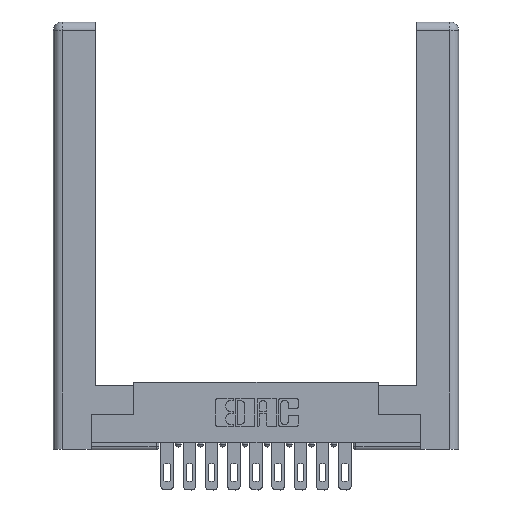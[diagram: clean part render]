
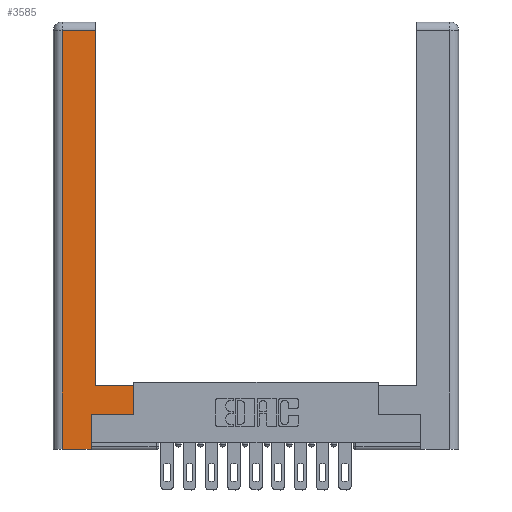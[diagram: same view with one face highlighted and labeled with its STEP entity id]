
A CAD part, top view. The second image highlights one B-rep face of the part: STEP entity #3585.
In plain terms, the highlighted planar face has unit normal (0, 0, 1).
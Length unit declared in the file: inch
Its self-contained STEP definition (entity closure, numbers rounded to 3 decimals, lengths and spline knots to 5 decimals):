
#285 = EDGE_CURVE ( 'NONE', #2528, #12402, #13260, .T. ) ;
#314 = VECTOR ( 'NONE', #14317, 39.37008 ) ;
#324 = DIRECTION ( 'NONE',  ( 0., -1., 0. ) ) ;
#341 = FACE_OUTER_BOUND ( 'NONE', #1421, .T. ) ;
#412 = EDGE_CURVE ( 'NONE', #4392, #11745, #2826, .T. ) ;
#579 = DIRECTION ( 'NONE',  ( -1., 0., 0. ) ) ;
#1043 = CARTESIAN_POINT ( 'NONE',  ( 0.565, 0.45, 0. ) ) ;
#1097 = CARTESIAN_POINT ( 'NONE',  ( 0.265, 0., 0. ) ) ;
#1421 = EDGE_LOOP ( 'NONE', ( #4682, #1939, #2007, #12526, #7499, #11966, #8899, #12150 ) ) ;
#1589 = CARTESIAN_POINT ( 'NONE',  ( 0.565, 0.245, 0. ) ) ;
#1939 = ORIENTED_EDGE ( 'NONE', *, *, #285, .T. ) ;
#2001 = CARTESIAN_POINT ( 'NONE',  ( 0.265, 0.245, 0. ) ) ;
#2007 = ORIENTED_EDGE ( 'NONE', *, *, #9992, .T. ) ;
#2528 = VERTEX_POINT ( 'NONE', #3374 ) ;
#2606 = VERTEX_POINT ( 'NONE', #13641 ) ;
#2651 = CARTESIAN_POINT ( 'NONE',  ( 0.295, 0.45, 0. ) ) ;
#2721 = VERTEX_POINT ( 'NONE', #9491 ) ;
#2760 = EDGE_CURVE ( 'NONE', #11745, #7623, #8735, .T. ) ;
#2802 = VECTOR ( 'NONE', #12551, 39.37008 ) ;
#2826 = LINE ( 'NONE', #7552, #11352 ) ;
#2842 = VECTOR ( 'NONE', #579, 39.37008 ) ;
#2878 = CARTESIAN_POINT ( 'NONE',  ( 0., 0., 0. ) ) ;
#2929 = CARTESIAN_POINT ( 'NONE',  ( 0.295, 3., 0. ) ) ;
#3374 = CARTESIAN_POINT ( 'NONE',  ( 0.295, 2.94, 0. ) ) ;
#3585 = ADVANCED_FACE ( 'NONE', ( #341 ), #11895, .F. ) ;
#4187 = VECTOR ( 'NONE', #324, 39.37008 ) ;
#4232 = EDGE_CURVE ( 'NONE', #9567, #2721, #6940, .T. ) ;
#4392 = VERTEX_POINT ( 'NONE', #8980 ) ;
#4682 = ORIENTED_EDGE ( 'NONE', *, *, #9092, .T. ) ;
#5014 = CARTESIAN_POINT ( 'NONE',  ( 0.0615, 0., 0. ) ) ;
#5118 = AXIS2_PLACEMENT_3D ( 'NONE', #2878, #5137, #5228 ) ;
#5137 = DIRECTION ( 'NONE',  ( 0., 0., -1. ) ) ;
#5228 = DIRECTION ( 'NONE',  ( -1., 0., 0. ) ) ;
#5252 = CARTESIAN_POINT ( 'NONE',  ( 0.295, 0.45, 0. ) ) ;
#5794 = VECTOR ( 'NONE', #7245, 39.37008 ) ;
#6509 = DIRECTION ( 'NONE',  ( 0., 1., 0. ) ) ;
#6940 = LINE ( 'NONE', #1097, #314 ) ;
#7245 = DIRECTION ( 'NONE',  ( -1., 0., 0. ) ) ;
#7499 = ORIENTED_EDGE ( 'NONE', *, *, #12125, .T. ) ;
#7552 = CARTESIAN_POINT ( 'NONE',  ( 0.565, 0.45, 0. ) ) ;
#7623 = VERTEX_POINT ( 'NONE', #5252 ) ;
#8471 = CARTESIAN_POINT ( 'NONE',  ( 0.0615, 2.94, 0. ) ) ;
#8722 = LINE ( 'NONE', #1589, #2802 ) ;
#8735 = LINE ( 'NONE', #2651, #5794 ) ;
#8899 = ORIENTED_EDGE ( 'NONE', *, *, #412, .T. ) ;
#8980 = CARTESIAN_POINT ( 'NONE',  ( 0.565, 0.245, 0. ) ) ;
#9092 = EDGE_CURVE ( 'NONE', #7623, #2528, #14120, .T. ) ;
#9491 = CARTESIAN_POINT ( 'NONE',  ( 0.265, 0., 0. ) ) ;
#9567 = VERTEX_POINT ( 'NONE', #5014 ) ;
#9928 = EDGE_CURVE ( 'NONE', #2606, #4392, #8722, .T. ) ;
#9992 = EDGE_CURVE ( 'NONE', #12402, #9567, #10487, .T. ) ;
#10378 = CARTESIAN_POINT ( 'NONE',  ( 0.0615, 0., 0. ) ) ;
#10487 = LINE ( 'NONE', #10378, #4187 ) ;
#11352 = VECTOR ( 'NONE', #14142, 39.37008 ) ;
#11745 = VERTEX_POINT ( 'NONE', #1043 ) ;
#11895 = PLANE ( 'NONE',  #5118 ) ;
#11966 = ORIENTED_EDGE ( 'NONE', *, *, #9928, .T. ) ;
#12057 = VECTOR ( 'NONE', #12091, 39.37008 ) ;
#12091 = DIRECTION ( 'NONE',  ( 0., 1., 0. ) ) ;
#12125 = EDGE_CURVE ( 'NONE', #2721, #2606, #12836, .T. ) ;
#12143 = VECTOR ( 'NONE', #6509, 39.37008 ) ;
#12150 = ORIENTED_EDGE ( 'NONE', *, *, #2760, .T. ) ;
#12402 = VERTEX_POINT ( 'NONE', #13724 ) ;
#12526 = ORIENTED_EDGE ( 'NONE', *, *, #4232, .T. ) ;
#12551 = DIRECTION ( 'NONE',  ( 1., 0., 0. ) ) ;
#12836 = LINE ( 'NONE', #2001, #12143 ) ;
#13260 = LINE ( 'NONE', #8471, #2842 ) ;
#13641 = CARTESIAN_POINT ( 'NONE',  ( 0.265, 0.245, 0. ) ) ;
#13724 = CARTESIAN_POINT ( 'NONE',  ( 0.0615, 2.94, 0. ) ) ;
#14120 = LINE ( 'NONE', #2929, #12057 ) ;
#14142 = DIRECTION ( 'NONE',  ( 0., 1., 0. ) ) ;
#14317 = DIRECTION ( 'NONE',  ( 1., 0., 0. ) ) ;
